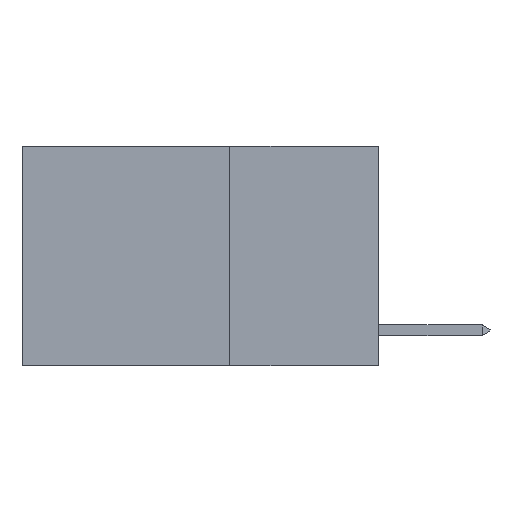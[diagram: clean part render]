
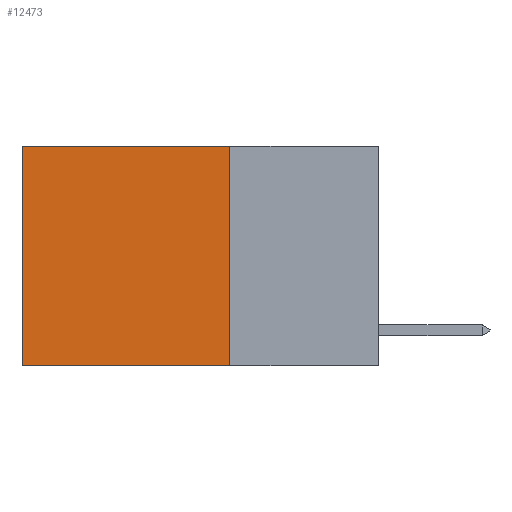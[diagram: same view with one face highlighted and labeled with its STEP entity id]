
A CAD part, left-side view. The second image highlights one B-rep face of the part: STEP entity #12473.
In plain terms, the highlighted planar face has unit normal (-1, 0, 0).
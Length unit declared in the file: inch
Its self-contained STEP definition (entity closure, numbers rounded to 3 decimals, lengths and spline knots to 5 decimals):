
#1070 = DIRECTION ( 'NONE',  ( 0., 1., 0. ) ) ;
#1264 = VECTOR ( 'NONE', #15868, 39.37008 ) ;
#1375 = ORIENTED_EDGE ( 'NONE', *, *, #9920, .F. ) ;
#1775 = CARTESIAN_POINT ( 'NONE',  ( 0.2625, 0.25, 0. ) ) ;
#2470 = CARTESIAN_POINT ( 'NONE',  ( 0.2625, 0.25, 0. ) ) ;
#2618 = DIRECTION ( 'NONE',  ( 0., 0., -1. ) ) ;
#2681 = VERTEX_POINT ( 'NONE', #13435 ) ;
#2722 = VECTOR ( 'NONE', #1070, 39.37008 ) ;
#3039 = VERTEX_POINT ( 'NONE', #2470 ) ;
#3041 = DIRECTION ( 'NONE',  ( 0., 1., 0. ) ) ;
#3295 = VECTOR ( 'NONE', #2618, 39.37008 ) ;
#4011 = VERTEX_POINT ( 'NONE', #13458 ) ;
#4911 = EDGE_CURVE ( 'NONE', #3039, #8825, #8258, .T. ) ;
#5035 = VECTOR ( 'NONE', #3041, 39.37008 ) ;
#5216 = DIRECTION ( 'NONE',  ( 0., 0., -1. ) ) ;
#5358 = CARTESIAN_POINT ( 'NONE',  ( 0.2625, 0.25, -0.37 ) ) ;
#5446 = LINE ( 'NONE', #1775, #5035 ) ;
#7467 = EDGE_CURVE ( 'NONE', #3039, #4011, #5446, .T. ) ;
#7746 = FACE_OUTER_BOUND ( 'NONE', #13588, .T. ) ;
#7785 = CARTESIAN_POINT ( 'NONE',  ( 0.2625, 0.25, 0. ) ) ;
#8258 = LINE ( 'NONE', #14594, #1264 ) ;
#8825 = VERTEX_POINT ( 'NONE', #5358 ) ;
#8955 = CARTESIAN_POINT ( 'NONE',  ( 0.2625, 0.25, -0.37 ) ) ;
#9875 = LINE ( 'NONE', #11779, #3295 ) ;
#9920 = EDGE_CURVE ( 'NONE', #8825, #2681, #14781, .T. ) ;
#10531 = EDGE_CURVE ( 'NONE', #4011, #2681, #9875, .T. ) ;
#11738 = PLANE ( 'NONE',  #15512 ) ;
#11779 = CARTESIAN_POINT ( 'NONE',  ( 0.2625, 0.6, 0. ) ) ;
#12473 = ADVANCED_FACE ( 'NONE', ( #7746 ), #11738, .F. ) ;
#13037 = DIRECTION ( 'NONE',  ( 1., 0., 0. ) ) ;
#13435 = CARTESIAN_POINT ( 'NONE',  ( 0.2625, 0.6, -0.37 ) ) ;
#13458 = CARTESIAN_POINT ( 'NONE',  ( 0.2625, 0.6, 0. ) ) ;
#13588 = EDGE_LOOP ( 'NONE', ( #15615, #1375, #16306, #14887 ) ) ;
#14594 = CARTESIAN_POINT ( 'NONE',  ( 0.2625, 0.25, 0. ) ) ;
#14781 = LINE ( 'NONE', #8955, #2722 ) ;
#14887 = ORIENTED_EDGE ( 'NONE', *, *, #7467, .T. ) ;
#15512 = AXIS2_PLACEMENT_3D ( 'NONE', #7785, #13037, #5216 ) ;
#15615 = ORIENTED_EDGE ( 'NONE', *, *, #10531, .T. ) ;
#15868 = DIRECTION ( 'NONE',  ( 0., 0., -1. ) ) ;
#16306 = ORIENTED_EDGE ( 'NONE', *, *, #4911, .F. ) ;
